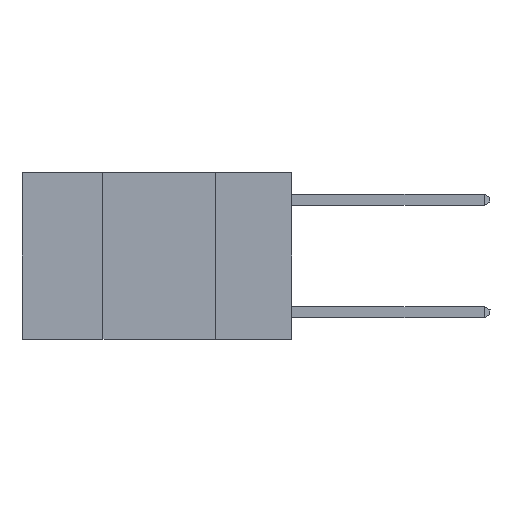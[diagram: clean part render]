
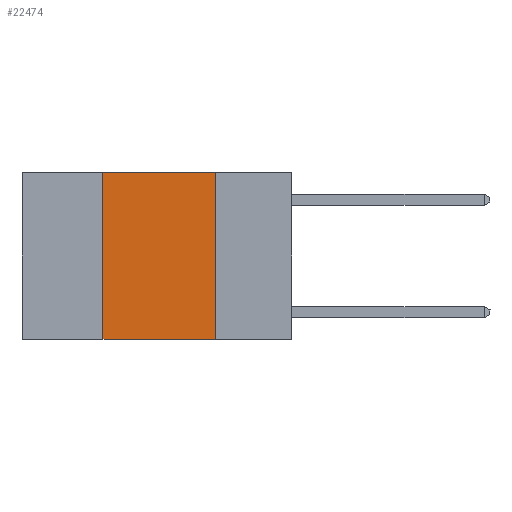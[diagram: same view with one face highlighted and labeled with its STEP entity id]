
A CAD part, left-side view. The second image highlights one B-rep face of the part: STEP entity #22474.
In plain terms, the highlighted planar face has unit normal (-1, 0, 0).
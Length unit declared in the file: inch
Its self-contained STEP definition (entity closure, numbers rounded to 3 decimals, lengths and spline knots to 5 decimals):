
#865 = EDGE_CURVE ( 'NONE', #12458, #21362, #28145, .T. ) ;
#1989 = CARTESIAN_POINT ( 'NONE',  ( 0., 0.6, 0. ) ) ;
#2277 = EDGE_LOOP ( 'NONE', ( #4937, #16199, #5715, #11385 ) ) ;
#4038 = LINE ( 'NONE', #6927, #16824 ) ;
#4504 = DIRECTION ( 'NONE',  ( 0., 0., -1. ) ) ;
#4937 = ORIENTED_EDGE ( 'NONE', *, *, #9071, .F. ) ;
#5146 = LINE ( 'NONE', #21941, #17147 ) ;
#5715 = ORIENTED_EDGE ( 'NONE', *, *, #865, .F. ) ;
#6927 = CARTESIAN_POINT ( 'NONE',  ( 0., 0.17, 0. ) ) ;
#8135 = VERTEX_POINT ( 'NONE', #29623 ) ;
#8853 = VERTEX_POINT ( 'NONE', #20535 ) ;
#8982 = DIRECTION ( 'NONE',  ( 0., -1., 0. ) ) ;
#9071 = EDGE_CURVE ( 'NONE', #8853, #8135, #4038, .T. ) ;
#11385 = ORIENTED_EDGE ( 'NONE', *, *, #26771, .T. ) ;
#12458 = VERTEX_POINT ( 'NONE', #22593 ) ;
#12461 = VECTOR ( 'NONE', #8982, 39.37008 ) ;
#13050 = CARTESIAN_POINT ( 'NONE',  ( 0., 0.42, 0. ) ) ;
#14081 = PLANE ( 'NONE',  #14802 ) ;
#14598 = EDGE_CURVE ( 'NONE', #21362, #8853, #18822, .T. ) ;
#14802 = AXIS2_PLACEMENT_3D ( 'NONE', #1989, #18899, #4504 ) ;
#16199 = ORIENTED_EDGE ( 'NONE', *, *, #14598, .F. ) ;
#16824 = VECTOR ( 'NONE', #23590, 39.37008 ) ;
#17147 = VECTOR ( 'NONE', #24333, 39.37008 ) ;
#18822 = LINE ( 'NONE', #20821, #12461 ) ;
#18899 = DIRECTION ( 'NONE',  ( 1., 0., 0. ) ) ;
#20535 = CARTESIAN_POINT ( 'NONE',  ( 0., 0.17, 0. ) ) ;
#20821 = CARTESIAN_POINT ( 'NONE',  ( 0., 0.6, 0. ) ) ;
#21362 = VERTEX_POINT ( 'NONE', #13050 ) ;
#21941 = CARTESIAN_POINT ( 'NONE',  ( 0., 0.6, -0.37 ) ) ;
#22474 = ADVANCED_FACE ( 'NONE', ( #24653 ), #14081, .F. ) ;
#22593 = CARTESIAN_POINT ( 'NONE',  ( 0., 0.42, -0.37 ) ) ;
#23590 = DIRECTION ( 'NONE',  ( 0., 0., -1. ) ) ;
#24333 = DIRECTION ( 'NONE',  ( 0., -1., 0. ) ) ;
#24653 = FACE_OUTER_BOUND ( 'NONE', #2277, .T. ) ;
#26771 = EDGE_CURVE ( 'NONE', #12458, #8135, #5146, .T. ) ;
#27285 = CARTESIAN_POINT ( 'NONE',  ( 0., 0.42, 0. ) ) ;
#27444 = VECTOR ( 'NONE', #30634, 39.37008 ) ;
#28145 = LINE ( 'NONE', #27285, #27444 ) ;
#29623 = CARTESIAN_POINT ( 'NONE',  ( 0., 0.17, -0.37 ) ) ;
#30634 = DIRECTION ( 'NONE',  ( 0., 0., 1. ) ) ;
